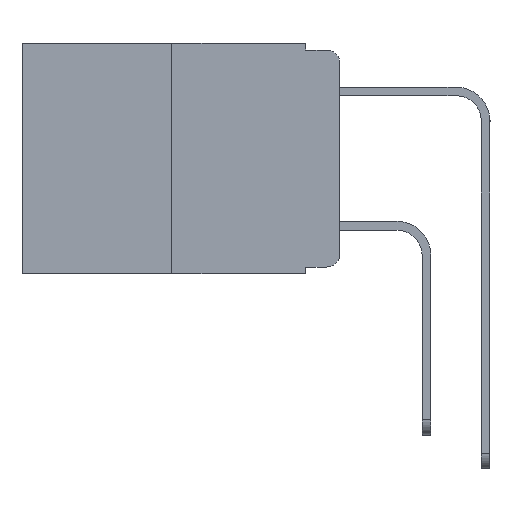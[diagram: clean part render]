
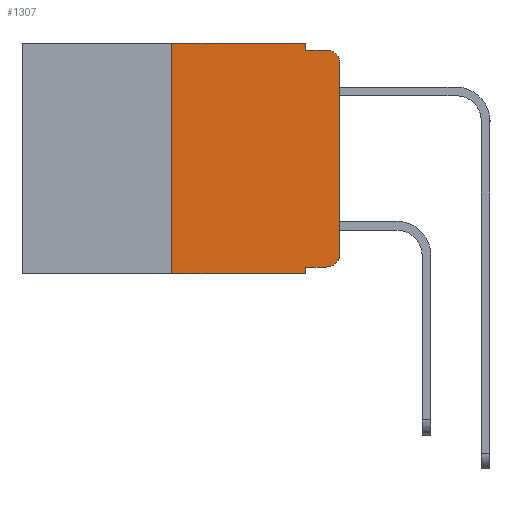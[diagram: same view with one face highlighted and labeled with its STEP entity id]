
A CAD part, left-side view. The second image highlights one B-rep face of the part: STEP entity #1307.
In plain terms, the highlighted planar face has unit normal (-1, 0, 0).
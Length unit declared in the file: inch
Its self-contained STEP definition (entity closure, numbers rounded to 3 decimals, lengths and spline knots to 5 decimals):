
#468 = EDGE_LOOP ( 'NONE', ( #865, #21406, #12112, #7765, #17676, #18251, #23110, #8953, #23673, #4530 ) ) ;
#788 = AXIS2_PLACEMENT_3D ( 'NONE', #9008, #21980, #10833 ) ;
#865 = ORIENTED_EDGE ( 'NONE', *, *, #12050, .T. ) ;
#1307 = ADVANCED_FACE ( 'NONE', ( #10092 ), #19666, .F. ) ;
#1314 = VECTOR ( 'NONE', #14799, 39.37008 ) ;
#1687 = CARTESIAN_POINT ( 'NONE',  ( 0., 0.25, -0.343 ) ) ;
#1714 = CARTESIAN_POINT ( 'NONE',  ( 0., 0.02, -0.03 ) ) ;
#1959 = LINE ( 'NONE', #21510, #5860 ) ;
#1960 = EDGE_CURVE ( 'NONE', #5399, #22356, #13272, .T. ) ;
#2905 = CARTESIAN_POINT ( 'NONE',  ( 0., 0.051, -0.333 ) ) ;
#2909 = LINE ( 'NONE', #11743, #7305 ) ;
#3284 = EDGE_CURVE ( 'NONE', #16788, #8030, #21998, .T. ) ;
#3412 = CARTESIAN_POINT ( 'NONE',  ( 0., 0.051, -0.343 ) ) ;
#3689 = DIRECTION ( 'NONE',  ( 0., 0., -1. ) ) ;
#4530 = ORIENTED_EDGE ( 'NONE', *, *, #11009, .T. ) ;
#4608 = CARTESIAN_POINT ( 'NONE',  ( 0., 0., -0.313 ) ) ;
#5031 = CIRCLE ( 'NONE', #788, 0.02 ) ;
#5399 = VERTEX_POINT ( 'NONE', #1687 ) ;
#5641 = EDGE_CURVE ( 'NONE', #18494, #8509, #14070, .T. ) ;
#5860 = VECTOR ( 'NONE', #16042, 39.37008 ) ;
#6236 = DIRECTION ( 'NONE',  ( 0., -1., 0. ) ) ;
#6330 = AXIS2_PLACEMENT_3D ( 'NONE', #1714, #14907, #3689 ) ;
#6793 = EDGE_CURVE ( 'NONE', #5399, #11036, #2909, .T. ) ;
#7064 = EDGE_CURVE ( 'NONE', #8030, #22377, #11361, .T. ) ;
#7305 = VECTOR ( 'NONE', #6236, 39.37008 ) ;
#7431 = DIRECTION ( 'NONE',  ( 0., 0., -1. ) ) ;
#7765 = ORIENTED_EDGE ( 'NONE', *, *, #3284, .F. ) ;
#8030 = VERTEX_POINT ( 'NONE', #12033 ) ;
#8349 = EDGE_CURVE ( 'NONE', #19134, #22377, #18631, .T. ) ;
#8509 = VERTEX_POINT ( 'NONE', #23269 ) ;
#8666 = DIRECTION ( 'NONE',  ( 0., 0., 1. ) ) ;
#8921 = VECTOR ( 'NONE', #8666, 39.37008 ) ;
#8953 = ORIENTED_EDGE ( 'NONE', *, *, #9393, .F. ) ;
#8981 = CARTESIAN_POINT ( 'NONE',  ( 0., 0.051, -0.333 ) ) ;
#9008 = CARTESIAN_POINT ( 'NONE',  ( 0., 0.02, -0.313 ) ) ;
#9199 = CARTESIAN_POINT ( 'NONE',  ( 0., 0., -0.03 ) ) ;
#9217 = VECTOR ( 'NONE', #17882, 39.37008 ) ;
#9393 = EDGE_CURVE ( 'NONE', #18494, #11036, #22240, .T. ) ;
#10092 = FACE_OUTER_BOUND ( 'NONE', #468, .T. ) ;
#10211 = VERTEX_POINT ( 'NONE', #4608 ) ;
#10541 = CARTESIAN_POINT ( 'NONE',  ( 0., 0.25, 0. ) ) ;
#10833 = DIRECTION ( 'NONE',  ( 0., 0., -1. ) ) ;
#11006 = CARTESIAN_POINT ( 'NONE',  ( 0., 0.051, -0.01 ) ) ;
#11009 = EDGE_CURVE ( 'NONE', #8509, #10211, #5031, .T. ) ;
#11036 = VERTEX_POINT ( 'NONE', #3412 ) ;
#11361 = LINE ( 'NONE', #11006, #1314 ) ;
#11743 = CARTESIAN_POINT ( 'NONE',  ( 0., 0.473, -0.343 ) ) ;
#11767 = VECTOR ( 'NONE', #7431, 39.37008 ) ;
#12033 = CARTESIAN_POINT ( 'NONE',  ( 0., 0.051, -0.01 ) ) ;
#12050 = EDGE_CURVE ( 'NONE', #10211, #19134, #1959, .T. ) ;
#12112 = ORIENTED_EDGE ( 'NONE', *, *, #7064, .F. ) ;
#12115 = VECTOR ( 'NONE', #12245, 39.37008 ) ;
#12245 = DIRECTION ( 'NONE',  ( 0., 0., -1. ) ) ;
#13272 = LINE ( 'NONE', #18185, #8921 ) ;
#14070 = LINE ( 'NONE', #2905, #14653 ) ;
#14423 = CARTESIAN_POINT ( 'NONE',  ( 0., 0.02, -0.01 ) ) ;
#14653 = VECTOR ( 'NONE', #16004, 39.37008 ) ;
#14799 = DIRECTION ( 'NONE',  ( 0., -1., 0. ) ) ;
#14868 = CARTESIAN_POINT ( 'NONE',  ( 0., 0.051, 0. ) ) ;
#14907 = DIRECTION ( 'NONE',  ( -1., 0., 0. ) ) ;
#15944 = CARTESIAN_POINT ( 'NONE',  ( 0., 0.473, 0. ) ) ;
#16004 = DIRECTION ( 'NONE',  ( 0., -1., 0. ) ) ;
#16042 = DIRECTION ( 'NONE',  ( 0., 0., 1. ) ) ;
#16788 = VERTEX_POINT ( 'NONE', #20687 ) ;
#17263 = DIRECTION ( 'NONE',  ( 0., 0., -1. ) ) ;
#17676 = ORIENTED_EDGE ( 'NONE', *, *, #17867, .F. ) ;
#17867 = EDGE_CURVE ( 'NONE', #22356, #16788, #19140, .T. ) ;
#17882 = DIRECTION ( 'NONE',  ( 0., -1., 0. ) ) ;
#18185 = CARTESIAN_POINT ( 'NONE',  ( 0., 0.25, 0. ) ) ;
#18251 = ORIENTED_EDGE ( 'NONE', *, *, #1960, .F. ) ;
#18494 = VERTEX_POINT ( 'NONE', #8981 ) ;
#18631 = CIRCLE ( 'NONE', #6330, 0.02 ) ;
#19134 = VERTEX_POINT ( 'NONE', #9199 ) ;
#19140 = LINE ( 'NONE', #15944, #9217 ) ;
#19208 = DIRECTION ( 'NONE',  ( 1., 0., 0. ) ) ;
#19666 = PLANE ( 'NONE',  #24021 ) ;
#20687 = CARTESIAN_POINT ( 'NONE',  ( 0., 0.051, 0. ) ) ;
#21406 = ORIENTED_EDGE ( 'NONE', *, *, #8349, .T. ) ;
#21492 = CARTESIAN_POINT ( 'NONE',  ( 0., 0.473, 0. ) ) ;
#21510 = CARTESIAN_POINT ( 'NONE',  ( 0., 0., 0. ) ) ;
#21980 = DIRECTION ( 'NONE',  ( -1., 0., 0. ) ) ;
#21998 = LINE ( 'NONE', #23329, #12115 ) ;
#22240 = LINE ( 'NONE', #14868, #11767 ) ;
#22356 = VERTEX_POINT ( 'NONE', #10541 ) ;
#22377 = VERTEX_POINT ( 'NONE', #14423 ) ;
#23110 = ORIENTED_EDGE ( 'NONE', *, *, #6793, .T. ) ;
#23269 = CARTESIAN_POINT ( 'NONE',  ( 0., 0.02, -0.333 ) ) ;
#23329 = CARTESIAN_POINT ( 'NONE',  ( 0., 0.051, 0. ) ) ;
#23673 = ORIENTED_EDGE ( 'NONE', *, *, #5641, .T. ) ;
#24021 = AXIS2_PLACEMENT_3D ( 'NONE', #21492, #19208, #17263 ) ;
